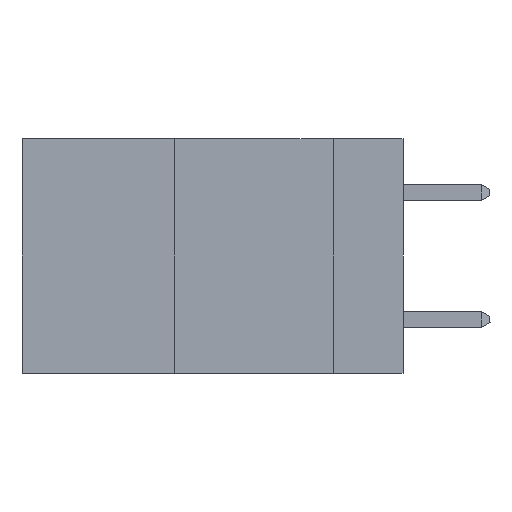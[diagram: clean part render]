
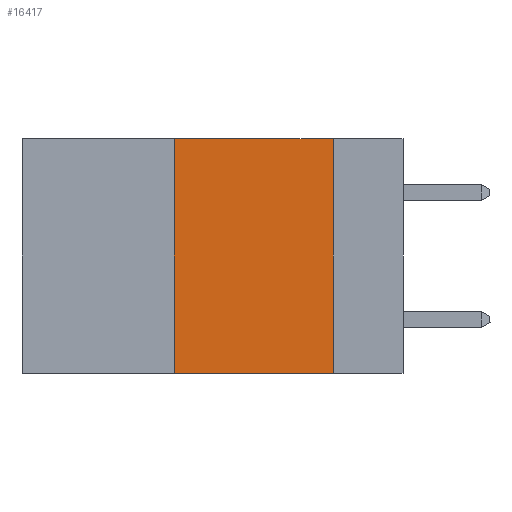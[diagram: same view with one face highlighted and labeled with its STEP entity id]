
A CAD part, left-side view. The second image highlights one B-rep face of the part: STEP entity #16417.
In plain terms, the highlighted planar face has unit normal (-1, 0, 0).
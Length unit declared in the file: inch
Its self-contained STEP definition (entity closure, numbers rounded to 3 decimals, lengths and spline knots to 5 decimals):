
#68 = FACE_OUTER_BOUND ( 'NONE', #2039, .T. ) ;
#976 = DIRECTION ( 'NONE',  ( 0., -1., 0. ) ) ;
#2039 = EDGE_LOOP ( 'NONE', ( #8630, #5796, #15362, #7284 ) ) ;
#2525 = DIRECTION ( 'NONE',  ( 0., 0., 1. ) ) ;
#3206 = VERTEX_POINT ( 'NONE', #12833 ) ;
#4377 = EDGE_CURVE ( 'NONE', #16311, #6444, #19211, .T. ) ;
#5152 = LINE ( 'NONE', #13581, #19920 ) ;
#5374 = VECTOR ( 'NONE', #22146, 39.37008 ) ;
#5796 = ORIENTED_EDGE ( 'NONE', *, *, #14889, .F. ) ;
#6239 = VERTEX_POINT ( 'NONE', #16597 ) ;
#6278 = VECTOR ( 'NONE', #976, 39.37008 ) ;
#6444 = VERTEX_POINT ( 'NONE', #7916 ) ;
#7284 = ORIENTED_EDGE ( 'NONE', *, *, #4377, .T. ) ;
#7848 = CARTESIAN_POINT ( 'NONE',  ( 0., 0.36, -0.37 ) ) ;
#7916 = CARTESIAN_POINT ( 'NONE',  ( 0., 0.11, -0.37 ) ) ;
#8155 = DIRECTION ( 'NONE',  ( 1., 0., 0. ) ) ;
#8630 = ORIENTED_EDGE ( 'NONE', *, *, #10542, .F. ) ;
#8857 = DIRECTION ( 'NONE',  ( 0., -1., 0. ) ) ;
#10542 = EDGE_CURVE ( 'NONE', #6239, #6444, #20158, .T. ) ;
#10760 = CARTESIAN_POINT ( 'NONE',  ( 0., 0.6, -0.37 ) ) ;
#11822 = AXIS2_PLACEMENT_3D ( 'NONE', #19327, #8155, #21260 ) ;
#12032 = CARTESIAN_POINT ( 'NONE',  ( 0., 0.6, 0. ) ) ;
#12833 = CARTESIAN_POINT ( 'NONE',  ( 0., 0.36, 0. ) ) ;
#13581 = CARTESIAN_POINT ( 'NONE',  ( 0., 0.36, 0. ) ) ;
#13705 = VECTOR ( 'NONE', #8857, 39.37008 ) ;
#14889 = EDGE_CURVE ( 'NONE', #3206, #6239, #15531, .T. ) ;
#15362 = ORIENTED_EDGE ( 'NONE', *, *, #19735, .F. ) ;
#15531 = LINE ( 'NONE', #12032, #6278 ) ;
#16311 = VERTEX_POINT ( 'NONE', #7848 ) ;
#16417 = ADVANCED_FACE ( 'NONE', ( #68 ), #17379, .F. ) ;
#16597 = CARTESIAN_POINT ( 'NONE',  ( 0., 0.11, 0. ) ) ;
#17379 = PLANE ( 'NONE',  #11822 ) ;
#19211 = LINE ( 'NONE', #10760, #13705 ) ;
#19327 = CARTESIAN_POINT ( 'NONE',  ( 0., 0.6, 0. ) ) ;
#19735 = EDGE_CURVE ( 'NONE', #16311, #3206, #5152, .T. ) ;
#19920 = VECTOR ( 'NONE', #2525, 39.37008 ) ;
#20158 = LINE ( 'NONE', #20260, #5374 ) ;
#20260 = CARTESIAN_POINT ( 'NONE',  ( 0., 0.11, 0. ) ) ;
#21260 = DIRECTION ( 'NONE',  ( 0., 0., -1. ) ) ;
#22146 = DIRECTION ( 'NONE',  ( 0., 0., -1. ) ) ;
